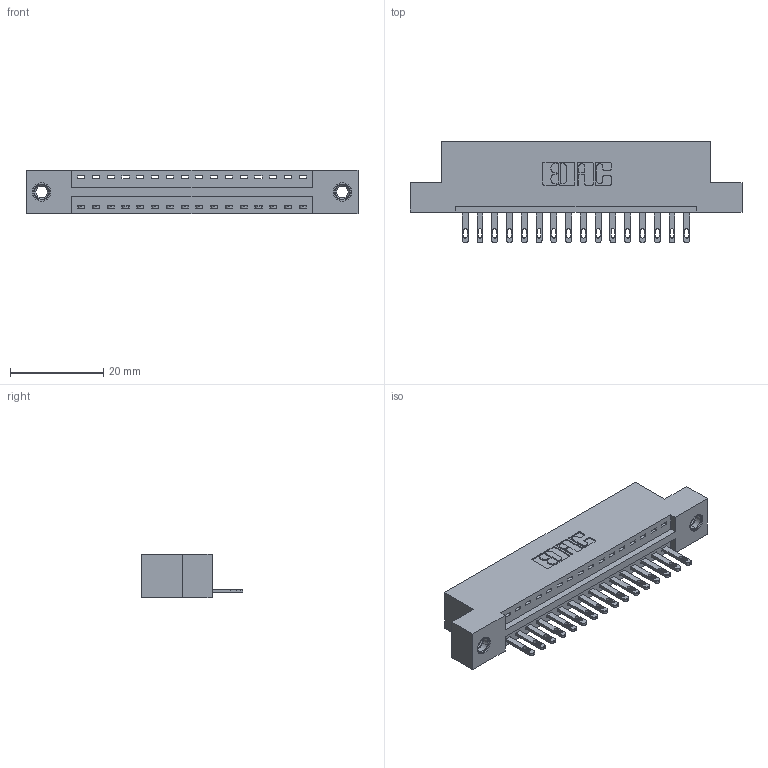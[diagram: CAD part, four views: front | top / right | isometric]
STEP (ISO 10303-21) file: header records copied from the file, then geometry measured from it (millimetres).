
FILE_DESCRIPTION (( 'STEP AP203' ), '1' );
FILE_NAME ('346-016-500-107.STEP', '2022-05-05T09:19:35', ( '' ), ( '' ), 'SwSTEP 2.0', 'SolidWorks 2020', '' );
FILE_SCHEMA (( 'CONFIG_CONTROL_DESIGN' ));
Length unit declared in the file: inch
Products named in the file (4): 346-016-500-107; 345-292-001_345-293-100; 345-250-001_345-250-005-103; 346 Part_Flush Mounting Lugs - 0.156 Dia-TI
Assembly tree (19 placements, depth 2):
  346-016-500-107
    346 Part_Flush Mounting Lugs - 0.156 Dia-TI
    345-292-001_345-293-100  x16
    345-250-001_345-250-005-103  x2
Bounding box: 71.37 x 21.84 x 9.4 mm (x, y, z)
Volume: 6649.3 mm3; surface area: 8102.2 mm2
Topology: 19 solids, 19 shells, 1046 faces, 3153 edges, 2094 vertices
Faces by surface type: plane 652, cylinder 378, cone 12, torus 4
Entity records: 14546 total; most frequent: CARTESIAN_POINT 2483, ORIENTED_EDGE 2426, DIRECTION 2251, EDGE_CURVE 1213, LINE 993, VECTOR 993, VERTEX_POINT 804, AXIS2_PLACEMENT_3D 629
